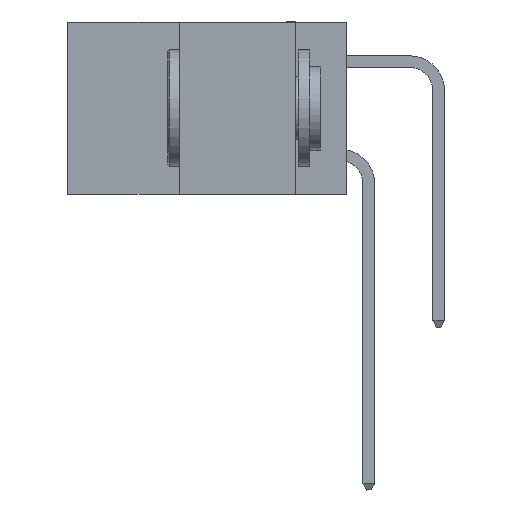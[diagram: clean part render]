
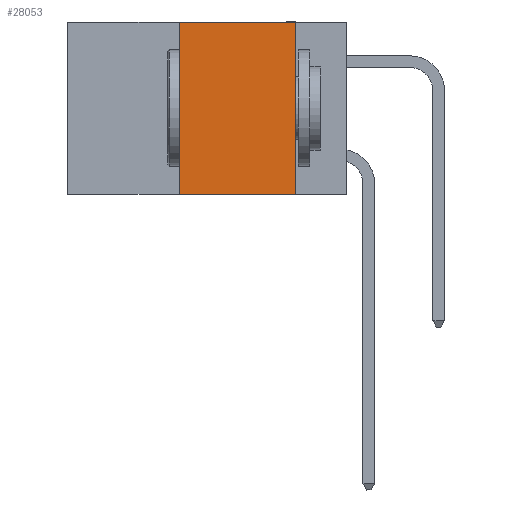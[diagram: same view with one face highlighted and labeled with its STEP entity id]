
A CAD part, left-side view. The second image highlights one B-rep face of the part: STEP entity #28053.
In plain terms, the highlighted planar face has unit normal (-1, 0, 0).
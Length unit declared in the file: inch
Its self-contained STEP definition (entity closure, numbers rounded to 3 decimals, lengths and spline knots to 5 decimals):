
#417 = EDGE_CURVE ( 'NONE', #17523, #20012, #18136, .T. ) ;
#626 = ORIENTED_EDGE ( 'NONE', *, *, #8542, .F. ) ;
#3707 = EDGE_CURVE ( 'NONE', #27714, #17659, #15865, .T. ) ;
#3909 = AXIS2_PLACEMENT_3D ( 'NONE', #21418, #32078, #16198 ) ;
#5127 = CARTESIAN_POINT ( 'NONE',  ( 0., 0.11, 0. ) ) ;
#5418 = DIRECTION ( 'NONE',  ( 0., -1., 0. ) ) ;
#5657 = CARTESIAN_POINT ( 'NONE',  ( 0., 0.6, -0.37 ) ) ;
#5883 = LINE ( 'NONE', #28035, #33456 ) ;
#6768 = DIRECTION ( 'NONE',  ( 0., 0., 1. ) ) ;
#8542 = EDGE_CURVE ( 'NONE', #27714, #17523, #5883, .T. ) ;
#8701 = VECTOR ( 'NONE', #5418, 39.37008 ) ;
#10979 = VECTOR ( 'NONE', #28982, 39.37008 ) ;
#12729 = DIRECTION ( 'NONE',  ( 0., 0., -1. ) ) ;
#12776 = CARTESIAN_POINT ( 'NONE',  ( 0., 0.6, 0. ) ) ;
#13340 = CARTESIAN_POINT ( 'NONE',  ( 0., 0.36, 0. ) ) ;
#13420 = ORIENTED_EDGE ( 'NONE', *, *, #19344, .F. ) ;
#13481 = PLANE ( 'NONE',  #3909 ) ;
#15865 = LINE ( 'NONE', #5657, #8701 ) ;
#16198 = DIRECTION ( 'NONE',  ( 0., 0., -1. ) ) ;
#17523 = VERTEX_POINT ( 'NONE', #13340 ) ;
#17659 = VERTEX_POINT ( 'NONE', #19308 ) ;
#18016 = CARTESIAN_POINT ( 'NONE',  ( 0., 0.11, 0. ) ) ;
#18136 = LINE ( 'NONE', #12776, #10979 ) ;
#19308 = CARTESIAN_POINT ( 'NONE',  ( 0., 0.11, -0.37 ) ) ;
#19344 = EDGE_CURVE ( 'NONE', #20012, #17659, #30060, .T. ) ;
#20012 = VERTEX_POINT ( 'NONE', #5127 ) ;
#21418 = CARTESIAN_POINT ( 'NONE',  ( 0., 0.6, 0. ) ) ;
#22204 = ORIENTED_EDGE ( 'NONE', *, *, #3707, .T. ) ;
#23040 = VECTOR ( 'NONE', #12729, 39.37008 ) ;
#27714 = VERTEX_POINT ( 'NONE', #28031 ) ;
#28031 = CARTESIAN_POINT ( 'NONE',  ( 0., 0.36, -0.37 ) ) ;
#28035 = CARTESIAN_POINT ( 'NONE',  ( 0., 0.36, 0. ) ) ;
#28053 = ADVANCED_FACE ( 'NONE', ( #32007 ), #13481, .F. ) ;
#28982 = DIRECTION ( 'NONE',  ( 0., -1., 0. ) ) ;
#30060 = LINE ( 'NONE', #18016, #23040 ) ;
#32007 = FACE_OUTER_BOUND ( 'NONE', #32135, .T. ) ;
#32078 = DIRECTION ( 'NONE',  ( 1., 0., 0. ) ) ;
#32135 = EDGE_LOOP ( 'NONE', ( #13420, #34630, #626, #22204 ) ) ;
#33456 = VECTOR ( 'NONE', #6768, 39.37008 ) ;
#34630 = ORIENTED_EDGE ( 'NONE', *, *, #417, .F. ) ;
